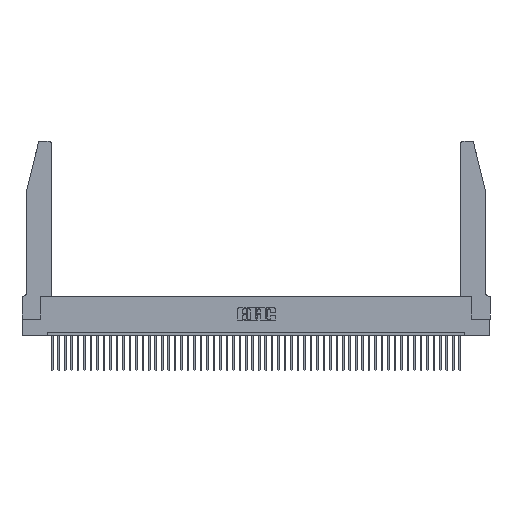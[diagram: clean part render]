
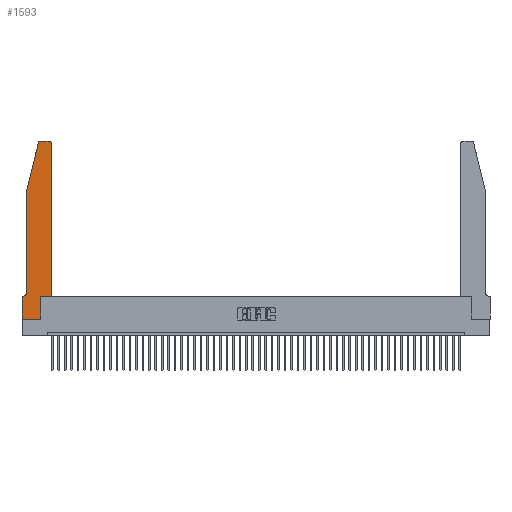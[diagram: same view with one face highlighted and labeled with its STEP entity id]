
A CAD part, top view. The second image highlights one B-rep face of the part: STEP entity #1593.
In plain terms, the highlighted planar face has unit normal (0, 0, 1).
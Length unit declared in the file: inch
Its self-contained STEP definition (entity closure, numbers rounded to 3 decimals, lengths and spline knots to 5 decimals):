
#658 = CARTESIAN_POINT ( 'NONE',  ( 0.284, 2.75, 0.37 ) ) ;
#1164 = CARTESIAN_POINT ( 'NONE',  ( 0.2605, 2.75, 0.37 ) ) ;
#1418 = CARTESIAN_POINT ( 'NONE',  ( 0.4505, 0.35, 0.37 ) ) ;
#1593 = ADVANCED_FACE ( 'NONE', ( #18216 ), #11078, .T. ) ;
#2045 = VERTEX_POINT ( 'NONE', #21006 ) ;
#2323 = EDGE_CURVE ( 'NONE', #19486, #3637, #23603, .T. ) ;
#3637 = VERTEX_POINT ( 'NONE', #17251 ) ;
#3977 = CIRCLE ( 'NONE', #34390, 0.03 ) ;
#4241 = DIRECTION ( 'NONE',  ( 0., 0., -1. ) ) ;
#5109 = LINE ( 'NONE', #43240, #44388 ) ;
#5189 = LINE ( 'NONE', #12286, #8785 ) ;
#5200 = CIRCLE ( 'NONE', #16072, 0.03 ) ;
#5340 = DIRECTION ( 'NONE',  ( 0., -1., 0. ) ) ;
#5731 = EDGE_CURVE ( 'NONE', #42842, #19571, #5200, .T. ) ;
#6430 = ORIENTED_EDGE ( 'NONE', *, *, #42577, .T. ) ;
#6483 = VERTEX_POINT ( 'NONE', #37420 ) ;
#7012 = CARTESIAN_POINT ( 'NONE',  ( 0.2865, 0., 0.37 ) ) ;
#7294 = ORIENTED_EDGE ( 'NONE', *, *, #21261, .T. ) ;
#7396 = DIRECTION ( 'NONE',  ( 0., 1., 0. ) ) ;
#7693 = ORIENTED_EDGE ( 'NONE', *, *, #2323, .T. ) ;
#7828 = DIRECTION ( 'NONE',  ( 0., -1., 0. ) ) ;
#8785 = VECTOR ( 'NONE', #27293, 39.37008 ) ;
#9035 = ORIENTED_EDGE ( 'NONE', *, *, #11956, .T. ) ;
#9714 = CARTESIAN_POINT ( 'NONE',  ( 0.4505, 2.72, 0.37 ) ) ;
#10436 = CARTESIAN_POINT ( 'NONE',  ( 0.0755, 0.42, 0.37 ) ) ;
#10586 = CARTESIAN_POINT ( 'NONE',  ( 0., 0.35, 0.37 ) ) ;
#11078 = PLANE ( 'NONE',  #34377 ) ;
#11151 = VECTOR ( 'NONE', #32772, 39.37008 ) ;
#11174 = ORIENTED_EDGE ( 'NONE', *, *, #33000, .T. ) ;
#11956 = EDGE_CURVE ( 'NONE', #40428, #46713, #5189, .T. ) ;
#12286 = CARTESIAN_POINT ( 'NONE',  ( 0., 0., 0.37 ) ) ;
#12719 = ORIENTED_EDGE ( 'NONE', *, *, #40471, .T. ) ;
#12949 = CARTESIAN_POINT ( 'NONE',  ( 0., 0., 0.37 ) ) ;
#13211 = EDGE_CURVE ( 'NONE', #3637, #36607, #47353, .T. ) ;
#13643 = DIRECTION ( 'NONE',  ( 1., 0., 0. ) ) ;
#15221 = VECTOR ( 'NONE', #7396, 39.37008 ) ;
#15862 = DIRECTION ( 'NONE',  ( 0., 0., 1. ) ) ;
#16072 = AXIS2_PLACEMENT_3D ( 'NONE', #44688, #32696, #13643 ) ;
#16148 = VERTEX_POINT ( 'NONE', #1418 ) ;
#16167 = LINE ( 'NONE', #30428, #31800 ) ;
#17251 = CARTESIAN_POINT ( 'NONE',  ( 0.0055, 0.35, 0.37 ) ) ;
#18100 = CARTESIAN_POINT ( 'NONE',  ( 0., 0.35, 0.37 ) ) ;
#18216 = FACE_OUTER_BOUND ( 'NONE', #21753, .T. ) ;
#19486 = VERTEX_POINT ( 'NONE', #10436 ) ;
#19571 = VERTEX_POINT ( 'NONE', #41930 ) ;
#19632 = DIRECTION ( 'NONE',  ( -1., 0., 0. ) ) ;
#21006 = CARTESIAN_POINT ( 'NONE',  ( 0.0755, 2., 0.37 ) ) ;
#21261 = EDGE_CURVE ( 'NONE', #6483, #16148, #37569, .T. ) ;
#21753 = EDGE_LOOP ( 'NONE', ( #23612, #42972, #25711, #23637, #7693, #32080, #39599, #9035, #11174, #7294, #6430, #12719 ) ) ;
#22888 = CARTESIAN_POINT ( 'NONE',  ( 0., 0., 0.37 ) ) ;
#23475 = DIRECTION ( 'NONE',  ( 1., 0., 0. ) ) ;
#23603 = CIRCLE ( 'NONE', #28222, 0.07 ) ;
#23612 = ORIENTED_EDGE ( 'NONE', *, *, #49123, .T. ) ;
#23637 = ORIENTED_EDGE ( 'NONE', *, *, #29689, .T. ) ;
#24816 = CARTESIAN_POINT ( 'NONE',  ( 0.4505, 0.35, 0.37 ) ) ;
#25711 = ORIENTED_EDGE ( 'NONE', *, *, #36355, .T. ) ;
#26932 = DIRECTION ( 'NONE',  ( 1., 0., 0. ) ) ;
#27293 = DIRECTION ( 'NONE',  ( 1., 0., 0. ) ) ;
#27567 = DIRECTION ( 'NONE',  ( 0., 1., 0. ) ) ;
#28222 = AXIS2_PLACEMENT_3D ( 'NONE', #39149, #4241, #19632 ) ;
#28227 = CARTESIAN_POINT ( 'NONE',  ( 0.0755, 0.35, 0.37 ) ) ;
#28500 = CARTESIAN_POINT ( 'NONE',  ( 0.4205, 2.75, 0.37 ) ) ;
#28900 = LINE ( 'NONE', #12949, #32522 ) ;
#29689 = EDGE_CURVE ( 'NONE', #2045, #19486, #16167, .T. ) ;
#30428 = CARTESIAN_POINT ( 'NONE',  ( 0.0755, 2., 0.37 ) ) ;
#30487 = CARTESIAN_POINT ( 'NONE',  ( 0.4205, 2.72, 0.37 ) ) ;
#31800 = VECTOR ( 'NONE', #7828, 39.37008 ) ;
#32080 = ORIENTED_EDGE ( 'NONE', *, *, #13211, .T. ) ;
#32522 = VECTOR ( 'NONE', #5340, 39.37008 ) ;
#32696 = DIRECTION ( 'NONE',  ( 0., 0., 1. ) ) ;
#32772 = DIRECTION ( 'NONE',  ( -1., 0., 0. ) ) ;
#33000 = EDGE_CURVE ( 'NONE', #46713, #6483, #5109, .T. ) ;
#33706 = DIRECTION ( 'NONE',  ( 1., 0., 0. ) ) ;
#34377 = AXIS2_PLACEMENT_3D ( 'NONE', #10586, #37732, #33706 ) ;
#34390 = AXIS2_PLACEMENT_3D ( 'NONE', #30487, #15862, #26932 ) ;
#35285 = LINE ( 'NONE', #1164, #42477 ) ;
#35513 = CARTESIAN_POINT ( 'NONE',  ( 0.4505, 0.35, 0.37 ) ) ;
#36355 = EDGE_CURVE ( 'NONE', #19571, #2045, #38605, .T. ) ;
#36607 = VERTEX_POINT ( 'NONE', #18100 ) ;
#36975 = VECTOR ( 'NONE', #23475, 39.37008 ) ;
#37008 = EDGE_CURVE ( 'NONE', #36607, #40428, #28900, .T. ) ;
#37420 = CARTESIAN_POINT ( 'NONE',  ( 0.2865, 0.35, 0.37 ) ) ;
#37569 = LINE ( 'NONE', #35513, #36975 ) ;
#37732 = DIRECTION ( 'NONE',  ( 0., 0., 1. ) ) ;
#38605 = LINE ( 'NONE', #39105, #42230 ) ;
#39105 = CARTESIAN_POINT ( 'NONE',  ( 0.0755, 2., 0.37 ) ) ;
#39149 = CARTESIAN_POINT ( 'NONE',  ( 0.0055, 0.42, 0.37 ) ) ;
#39599 = ORIENTED_EDGE ( 'NONE', *, *, #37008, .T. ) ;
#40428 = VERTEX_POINT ( 'NONE', #22888 ) ;
#40471 = EDGE_CURVE ( 'NONE', #48515, #41957, #3977, .T. ) ;
#41930 = CARTESIAN_POINT ( 'NONE',  ( 0.25487, 2.72718, 0.37 ) ) ;
#41957 = VERTEX_POINT ( 'NONE', #28500 ) ;
#42230 = VECTOR ( 'NONE', #46880, 39.37008 ) ;
#42477 = VECTOR ( 'NONE', #43000, 39.37008 ) ;
#42577 = EDGE_CURVE ( 'NONE', #16148, #48515, #45983, .T. ) ;
#42842 = VERTEX_POINT ( 'NONE', #658 ) ;
#42972 = ORIENTED_EDGE ( 'NONE', *, *, #5731, .T. ) ;
#43000 = DIRECTION ( 'NONE',  ( -1., 0., 0. ) ) ;
#43240 = CARTESIAN_POINT ( 'NONE',  ( 0.2865, 0.35, 0.37 ) ) ;
#44388 = VECTOR ( 'NONE', #27567, 39.37008 ) ;
#44688 = CARTESIAN_POINT ( 'NONE',  ( 0.284, 2.72, 0.37 ) ) ;
#45983 = LINE ( 'NONE', #24816, #15221 ) ;
#46713 = VERTEX_POINT ( 'NONE', #7012 ) ;
#46880 = DIRECTION ( 'NONE',  ( -0.239, -0.971, 0. ) ) ;
#47353 = LINE ( 'NONE', #28227, #11151 ) ;
#48515 = VERTEX_POINT ( 'NONE', #9714 ) ;
#49123 = EDGE_CURVE ( 'NONE', #41957, #42842, #35285, .T. ) ;
